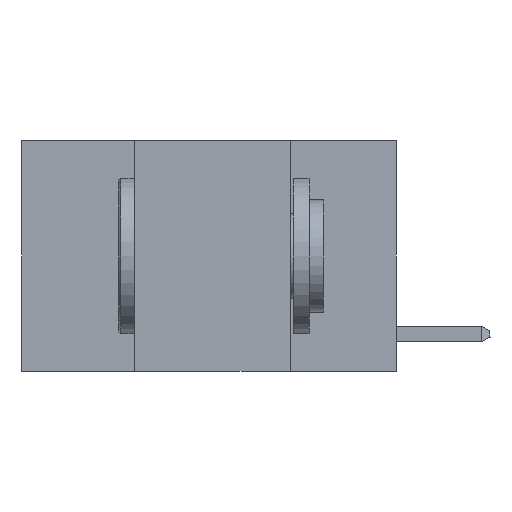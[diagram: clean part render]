
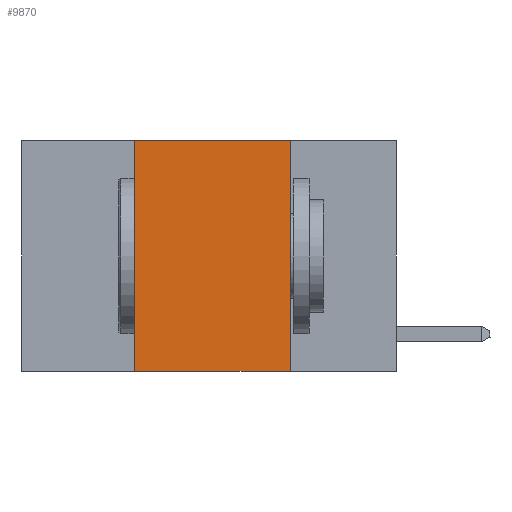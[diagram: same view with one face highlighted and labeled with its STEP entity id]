
A CAD part, left-side view. The second image highlights one B-rep face of the part: STEP entity #9870.
In plain terms, the highlighted planar face has unit normal (-1, 0, 0).
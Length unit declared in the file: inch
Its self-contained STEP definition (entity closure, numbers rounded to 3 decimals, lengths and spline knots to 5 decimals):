
#435 = CARTESIAN_POINT ( 'NONE',  ( 0., 0.6, 0. ) ) ;
#660 = CARTESIAN_POINT ( 'NONE',  ( 0., 0.6, -0.37 ) ) ;
#1150 = LINE ( 'NONE', #4294, #7716 ) ;
#1512 = CARTESIAN_POINT ( 'NONE',  ( 0., 0.6, 0. ) ) ;
#1759 = FACE_OUTER_BOUND ( 'NONE', #13871, .T. ) ;
#3117 = PLANE ( 'NONE',  #15630 ) ;
#3769 = EDGE_CURVE ( 'NONE', #14089, #6995, #6262, .T. ) ;
#4174 = DIRECTION ( 'NONE',  ( 0., -1., 0. ) ) ;
#4294 = CARTESIAN_POINT ( 'NONE',  ( 0., 0.17, 0. ) ) ;
#4425 = DIRECTION ( 'NONE',  ( 0., 0., -1. ) ) ;
#4632 = DIRECTION ( 'NONE',  ( 0., -1., 0. ) ) ;
#6262 = LINE ( 'NONE', #660, #9298 ) ;
#6897 = EDGE_CURVE ( 'NONE', #10616, #10775, #16112, .T. ) ;
#6995 = VERTEX_POINT ( 'NONE', #13431 ) ;
#7565 = CARTESIAN_POINT ( 'NONE',  ( 0., 0.17, 0. ) ) ;
#7716 = VECTOR ( 'NONE', #14583, 39.37008 ) ;
#8086 = LINE ( 'NONE', #10547, #14496 ) ;
#9298 = VECTOR ( 'NONE', #4632, 39.37008 ) ;
#9676 = EDGE_CURVE ( 'NONE', #14089, #10616, #8086, .T. ) ;
#9870 = ADVANCED_FACE ( 'NONE', ( #1759 ), #3117, .F. ) ;
#10547 = CARTESIAN_POINT ( 'NONE',  ( 0., 0.42, 0. ) ) ;
#10616 = VERTEX_POINT ( 'NONE', #16163 ) ;
#10775 = VERTEX_POINT ( 'NONE', #7565 ) ;
#11112 = ORIENTED_EDGE ( 'NONE', *, *, #6897, .F. ) ;
#11254 = ORIENTED_EDGE ( 'NONE', *, *, #3769, .T. ) ;
#11856 = DIRECTION ( 'NONE',  ( 0., 0., 1. ) ) ;
#12021 = ORIENTED_EDGE ( 'NONE', *, *, #15707, .F. ) ;
#12072 = ORIENTED_EDGE ( 'NONE', *, *, #9676, .F. ) ;
#12191 = DIRECTION ( 'NONE',  ( 1., 0., 0. ) ) ;
#12438 = VECTOR ( 'NONE', #4174, 39.37008 ) ;
#12563 = CARTESIAN_POINT ( 'NONE',  ( 0., 0.42, -0.37 ) ) ;
#13431 = CARTESIAN_POINT ( 'NONE',  ( 0., 0.17, -0.37 ) ) ;
#13871 = EDGE_LOOP ( 'NONE', ( #12021, #11112, #12072, #11254 ) ) ;
#14089 = VERTEX_POINT ( 'NONE', #12563 ) ;
#14496 = VECTOR ( 'NONE', #11856, 39.37008 ) ;
#14583 = DIRECTION ( 'NONE',  ( 0., 0., -1. ) ) ;
#15630 = AXIS2_PLACEMENT_3D ( 'NONE', #435, #12191, #4425 ) ;
#15707 = EDGE_CURVE ( 'NONE', #10775, #6995, #1150, .T. ) ;
#16112 = LINE ( 'NONE', #1512, #12438 ) ;
#16163 = CARTESIAN_POINT ( 'NONE',  ( 0., 0.42, 0. ) ) ;
